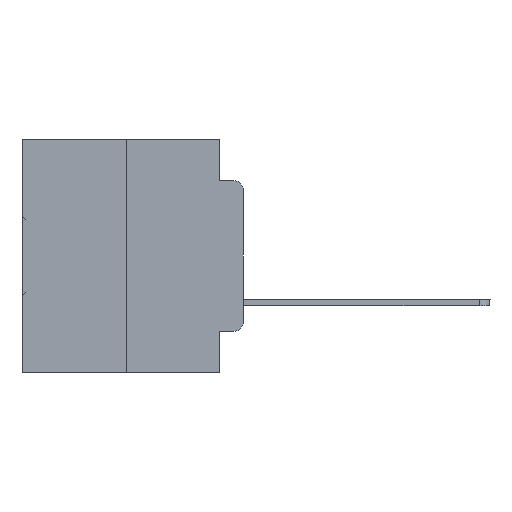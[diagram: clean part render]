
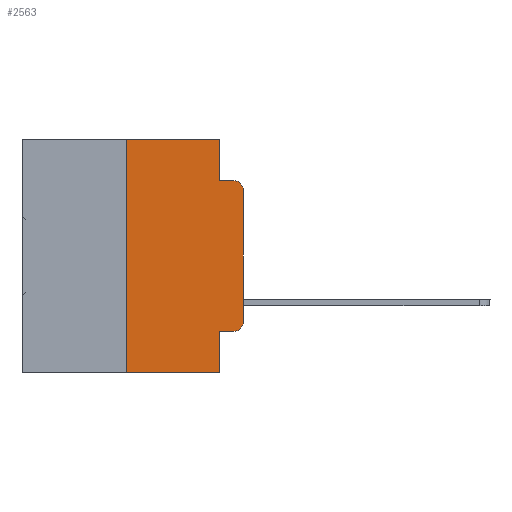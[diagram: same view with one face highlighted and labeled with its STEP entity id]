
A CAD part, left-side view. The second image highlights one B-rep face of the part: STEP entity #2563.
In plain terms, the highlighted planar face has unit normal (-1, 0, 0).
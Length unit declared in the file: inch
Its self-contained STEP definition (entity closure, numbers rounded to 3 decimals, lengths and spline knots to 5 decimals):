
#626 = DIRECTION ( 'NONE',  ( 0., 0., -1. ) ) ;
#688 = FACE_OUTER_BOUND ( 'NONE', #10075, .T. ) ;
#1271 = AXIS2_PLACEMENT_3D ( 'NONE', #29749, #20140, #14854 ) ;
#1449 = LINE ( 'NONE', #18066, #4605 ) ;
#1558 = CARTESIAN_POINT ( 'NONE',  ( 0., 0., 0. ) ) ;
#1829 = ORIENTED_EDGE ( 'NONE', *, *, #21729, .F. ) ;
#2190 = VERTEX_POINT ( 'NONE', #10966 ) ;
#2563 = ADVANCED_FACE ( 'NONE', ( #688 ), #30037, .F. ) ;
#2688 = DIRECTION ( 'NONE',  ( 0., 0., -1. ) ) ;
#4605 = VECTOR ( 'NONE', #626, 39.37008 ) ;
#5118 = VERTEX_POINT ( 'NONE', #24665 ) ;
#5334 = VECTOR ( 'NONE', #6628, 39.37008 ) ;
#5438 = ORIENTED_EDGE ( 'NONE', *, *, #23541, .F. ) ;
#5702 = VECTOR ( 'NONE', #21994, 39.37008 ) ;
#5988 = AXIS2_PLACEMENT_3D ( 'NONE', #7968, #15168, #2688 ) ;
#6328 = LINE ( 'NONE', #31240, #17946 ) ;
#6628 = DIRECTION ( 'NONE',  ( 0., 0., 1. ) ) ;
#7277 = VERTEX_POINT ( 'NONE', #15462 ) ;
#7353 = EDGE_CURVE ( 'NONE', #11221, #5118, #6328, .T. ) ;
#7370 = ORIENTED_EDGE ( 'NONE', *, *, #28025, .F. ) ;
#7968 = CARTESIAN_POINT ( 'NONE',  ( 0., 0.473, 0. ) ) ;
#8383 = EDGE_CURVE ( 'NONE', #2190, #23492, #31554, .T. ) ;
#8775 = CARTESIAN_POINT ( 'NONE',  ( 0., 0.051, -0.4115 ) ) ;
#9151 = CARTESIAN_POINT ( 'NONE',  ( 0., 0.02, -0.3915 ) ) ;
#9876 = CARTESIAN_POINT ( 'NONE',  ( 0., 0.473, -0.5 ) ) ;
#10075 = EDGE_LOOP ( 'NONE', ( #30942, #14678, #1829, #23316, #5438, #14199, #29760, #7370, #26643, #28513 ) ) ;
#10409 = CIRCLE ( 'NONE', #1271, 0.02 ) ;
#10966 = CARTESIAN_POINT ( 'NONE',  ( 0., 0.25, -0.5 ) ) ;
#11221 = VERTEX_POINT ( 'NONE', #14612 ) ;
#11595 = VERTEX_POINT ( 'NONE', #26322 ) ;
#12029 = CARTESIAN_POINT ( 'NONE',  ( 0., 0.25, 0. ) ) ;
#13228 = VERTEX_POINT ( 'NONE', #13856 ) ;
#13739 = DIRECTION ( 'NONE',  ( 0., 0., -1. ) ) ;
#13856 = CARTESIAN_POINT ( 'NONE',  ( 0., 0.02, -0.0885 ) ) ;
#14196 = LINE ( 'NONE', #12029, #24995 ) ;
#14199 = ORIENTED_EDGE ( 'NONE', *, *, #31957, .F. ) ;
#14382 = VERTEX_POINT ( 'NONE', #18127 ) ;
#14612 = CARTESIAN_POINT ( 'NONE',  ( 0., 0.051, 0. ) ) ;
#14678 = ORIENTED_EDGE ( 'NONE', *, *, #22904, .T. ) ;
#14854 = DIRECTION ( 'NONE',  ( 0., 0., -1. ) ) ;
#15168 = DIRECTION ( 'NONE',  ( 1., 0., 0. ) ) ;
#15462 = CARTESIAN_POINT ( 'NONE',  ( 0., 0.051, -0.4115 ) ) ;
#15512 = VECTOR ( 'NONE', #24188, 39.37008 ) ;
#17940 = DIRECTION ( 'NONE',  ( 0., 0., 1. ) ) ;
#17946 = VECTOR ( 'NONE', #13739, 39.37008 ) ;
#18066 = CARTESIAN_POINT ( 'NONE',  ( 0., 0.051, 0. ) ) ;
#18127 = CARTESIAN_POINT ( 'NONE',  ( 0., 0.25, 0. ) ) ;
#18264 = EDGE_CURVE ( 'NONE', #11595, #31738, #19351, .T. ) ;
#19088 = CARTESIAN_POINT ( 'NONE',  ( 0., 0., -0.1085 ) ) ;
#19351 = LINE ( 'NONE', #1558, #5334 ) ;
#19373 = DIRECTION ( 'NONE',  ( 0., -1., 0. ) ) ;
#19470 = LINE ( 'NONE', #24037, #22920 ) ;
#20140 = DIRECTION ( 'NONE',  ( -1., 0., 0. ) ) ;
#20286 = CARTESIAN_POINT ( 'NONE',  ( 0., 0.02, -0.4115 ) ) ;
#21674 = LINE ( 'NONE', #31923, #5702 ) ;
#21729 = EDGE_CURVE ( 'NONE', #5118, #13228, #19470, .T. ) ;
#21739 = LINE ( 'NONE', #8775, #15512 ) ;
#21994 = DIRECTION ( 'NONE',  ( 0., -1., 0. ) ) ;
#22588 = EDGE_CURVE ( 'NONE', #7277, #27335, #21739, .T. ) ;
#22904 = EDGE_CURVE ( 'NONE', #31738, #13228, #10409, .T. ) ;
#22920 = VECTOR ( 'NONE', #19373, 39.37008 ) ;
#23316 = ORIENTED_EDGE ( 'NONE', *, *, #7353, .F. ) ;
#23492 = VERTEX_POINT ( 'NONE', #32230 ) ;
#23541 = EDGE_CURVE ( 'NONE', #14382, #11221, #21674, .T. ) ;
#23829 = AXIS2_PLACEMENT_3D ( 'NONE', #9151, #24111, #32191 ) ;
#24037 = CARTESIAN_POINT ( 'NONE',  ( 0., 0.051, -0.0885 ) ) ;
#24087 = EDGE_CURVE ( 'NONE', #27335, #11595, #27437, .T. ) ;
#24111 = DIRECTION ( 'NONE',  ( -1., 0., 0. ) ) ;
#24188 = DIRECTION ( 'NONE',  ( 0., -1., 0. ) ) ;
#24304 = DIRECTION ( 'NONE',  ( 0., -1., 0. ) ) ;
#24665 = CARTESIAN_POINT ( 'NONE',  ( 0., 0.051, -0.0885 ) ) ;
#24995 = VECTOR ( 'NONE', #17940, 39.37008 ) ;
#26322 = CARTESIAN_POINT ( 'NONE',  ( 0., 0., -0.3915 ) ) ;
#26643 = ORIENTED_EDGE ( 'NONE', *, *, #22588, .T. ) ;
#27335 = VERTEX_POINT ( 'NONE', #20286 ) ;
#27437 = CIRCLE ( 'NONE', #23829, 0.02 ) ;
#28025 = EDGE_CURVE ( 'NONE', #7277, #23492, #1449, .T. ) ;
#28513 = ORIENTED_EDGE ( 'NONE', *, *, #24087, .T. ) ;
#29749 = CARTESIAN_POINT ( 'NONE',  ( 0., 0.02, -0.1085 ) ) ;
#29760 = ORIENTED_EDGE ( 'NONE', *, *, #8383, .T. ) ;
#30037 = PLANE ( 'NONE',  #5988 ) ;
#30728 = VECTOR ( 'NONE', #24304, 39.37008 ) ;
#30942 = ORIENTED_EDGE ( 'NONE', *, *, #18264, .T. ) ;
#31240 = CARTESIAN_POINT ( 'NONE',  ( 0., 0.051, 0. ) ) ;
#31554 = LINE ( 'NONE', #9876, #30728 ) ;
#31738 = VERTEX_POINT ( 'NONE', #19088 ) ;
#31923 = CARTESIAN_POINT ( 'NONE',  ( 0., 0.473, 0. ) ) ;
#31957 = EDGE_CURVE ( 'NONE', #2190, #14382, #14196, .T. ) ;
#32191 = DIRECTION ( 'NONE',  ( 0., 0., -1. ) ) ;
#32230 = CARTESIAN_POINT ( 'NONE',  ( 0., 0.051, -0.5 ) ) ;
